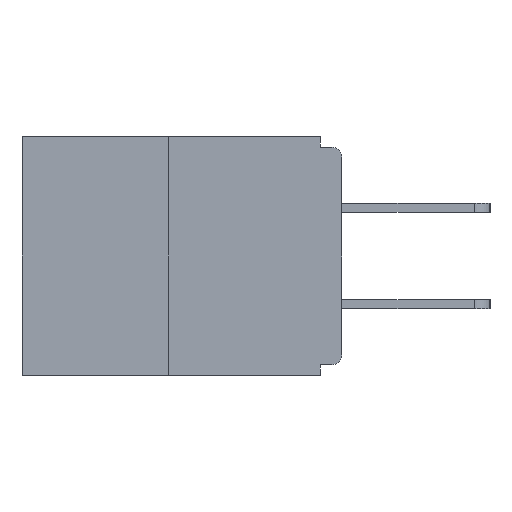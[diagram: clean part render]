
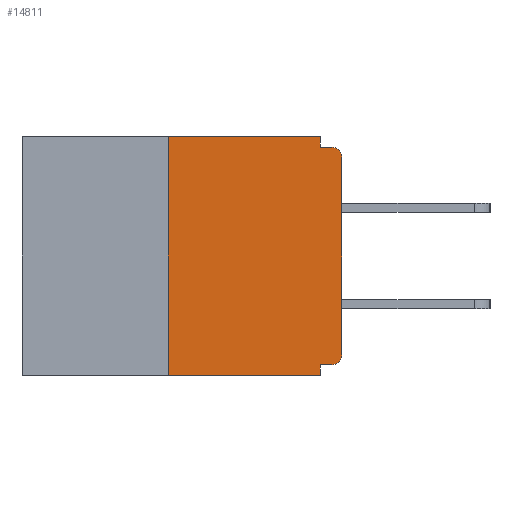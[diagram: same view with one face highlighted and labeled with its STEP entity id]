
A CAD part, left-side view. The second image highlights one B-rep face of the part: STEP entity #14811.
In plain terms, the highlighted planar face has unit normal (-1, 0, 0).
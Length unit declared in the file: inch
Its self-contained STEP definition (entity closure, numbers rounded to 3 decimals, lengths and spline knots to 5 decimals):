
#341 = EDGE_CURVE ( 'NONE', #14174, #8552, #1173, .T. ) ;
#707 = DIRECTION ( 'NONE',  ( 0., -1., 0. ) ) ;
#880 = ORIENTED_EDGE ( 'NONE', *, *, #341, .T. ) ;
#1102 = CARTESIAN_POINT ( 'NONE',  ( 0., 0.46, 0. ) ) ;
#1124 = DIRECTION ( 'NONE',  ( -1., 0., 0. ) ) ;
#1173 = CIRCLE ( 'NONE', #8427, 0.015 ) ;
#1279 = CIRCLE ( 'NONE', #10264, 0.015 ) ;
#1288 = ORIENTED_EDGE ( 'NONE', *, *, #7465, .T. ) ;
#2062 = CARTESIAN_POINT ( 'NONE',  ( 0., 0.25, 0. ) ) ;
#2180 = DIRECTION ( 'NONE',  ( 0., 0., -1. ) ) ;
#2292 = CARTESIAN_POINT ( 'NONE',  ( 0., 0.46, 0. ) ) ;
#2554 = CARTESIAN_POINT ( 'NONE',  ( 0., 0., 0. ) ) ;
#2937 = CARTESIAN_POINT ( 'NONE',  ( 0., 0.031, 0. ) ) ;
#3045 = LINE ( 'NONE', #2554, #7253 ) ;
#3136 = CARTESIAN_POINT ( 'NONE',  ( 0., 0.46, -0.343 ) ) ;
#3479 = LINE ( 'NONE', #16419, #13232 ) ;
#3625 = CARTESIAN_POINT ( 'NONE',  ( 0., 0.015, -0.015 ) ) ;
#3666 = DIRECTION ( 'NONE',  ( 0., 0., -1. ) ) ;
#3782 = CARTESIAN_POINT ( 'NONE',  ( 0., 0.015, -0.313 ) ) ;
#3856 = DIRECTION ( 'NONE',  ( 0., 0., 1. ) ) ;
#3902 = VERTEX_POINT ( 'NONE', #15123 ) ;
#4076 = EDGE_CURVE ( 'NONE', #8960, #9336, #14399, .T. ) ;
#4506 = DIRECTION ( 'NONE',  ( 0., -1., 0. ) ) ;
#4592 = EDGE_CURVE ( 'NONE', #7053, #8552, #11585, .T. ) ;
#4997 = PLANE ( 'NONE',  #16211 ) ;
#5063 = FACE_OUTER_BOUND ( 'NONE', #15114, .T. ) ;
#5150 = VERTEX_POINT ( 'NONE', #14991 ) ;
#5165 = CARTESIAN_POINT ( 'NONE',  ( 0., 0.25, 0. ) ) ;
#5410 = EDGE_CURVE ( 'NONE', #5150, #14174, #3045, .T. ) ;
#5808 = EDGE_CURVE ( 'NONE', #12360, #8960, #14711, .T. ) ;
#5948 = VERTEX_POINT ( 'NONE', #15202 ) ;
#6008 = CARTESIAN_POINT ( 'NONE',  ( 0., 0., -0.328 ) ) ;
#6629 = VERTEX_POINT ( 'NONE', #14404 ) ;
#6917 = EDGE_CURVE ( 'NONE', #6629, #3902, #3479, .T. ) ;
#7018 = EDGE_CURVE ( 'NONE', #5948, #5150, #1279, .T. ) ;
#7053 = VERTEX_POINT ( 'NONE', #7531 ) ;
#7224 = EDGE_CURVE ( 'NONE', #9336, #7053, #13584, .T. ) ;
#7253 = VECTOR ( 'NONE', #3856, 39.37008 ) ;
#7378 = DIRECTION ( 'NONE',  ( 0., 1., 0. ) ) ;
#7448 = CARTESIAN_POINT ( 'NONE',  ( 0., 0., -0.03 ) ) ;
#7465 = EDGE_CURVE ( 'NONE', #12360, #3902, #15368, .T. ) ;
#7504 = VECTOR ( 'NONE', #14130, 39.37008 ) ;
#7531 = CARTESIAN_POINT ( 'NONE',  ( 0., 0.031, -0.015 ) ) ;
#7771 = ORIENTED_EDGE ( 'NONE', *, *, #7018, .T. ) ;
#7797 = ORIENTED_EDGE ( 'NONE', *, *, #7224, .F. ) ;
#8427 = AXIS2_PLACEMENT_3D ( 'NONE', #12504, #1124, #2180 ) ;
#8552 = VERTEX_POINT ( 'NONE', #3625 ) ;
#8960 = VERTEX_POINT ( 'NONE', #5165 ) ;
#9336 = VERTEX_POINT ( 'NONE', #2937 ) ;
#9539 = VECTOR ( 'NONE', #707, 39.37008 ) ;
#9645 = CARTESIAN_POINT ( 'NONE',  ( 0., 0., -0.015 ) ) ;
#9994 = ORIENTED_EDGE ( 'NONE', *, *, #6917, .F. ) ;
#10100 = CARTESIAN_POINT ( 'NONE',  ( 0., 0.25, -0.343 ) ) ;
#10264 = AXIS2_PLACEMENT_3D ( 'NONE', #3782, #15272, #12943 ) ;
#11237 = DIRECTION ( 'NONE',  ( 0., 0., -1. ) ) ;
#11585 = LINE ( 'NONE', #9645, #13567 ) ;
#12360 = VERTEX_POINT ( 'NONE', #10100 ) ;
#12504 = CARTESIAN_POINT ( 'NONE',  ( 0., 0.015, -0.03 ) ) ;
#12943 = DIRECTION ( 'NONE',  ( 0., 0., -1. ) ) ;
#13232 = VECTOR ( 'NONE', #11237, 39.37008 ) ;
#13520 = VECTOR ( 'NONE', #14925, 39.37008 ) ;
#13547 = LINE ( 'NONE', #6008, #16379 ) ;
#13567 = VECTOR ( 'NONE', #4506, 39.37008 ) ;
#13584 = LINE ( 'NONE', #14018, #15382 ) ;
#14018 = CARTESIAN_POINT ( 'NONE',  ( 0., 0.031, 0. ) ) ;
#14130 = DIRECTION ( 'NONE',  ( 0., -1., 0. ) ) ;
#14174 = VERTEX_POINT ( 'NONE', #7448 ) ;
#14197 = ORIENTED_EDGE ( 'NONE', *, *, #5808, .F. ) ;
#14399 = LINE ( 'NONE', #1102, #7504 ) ;
#14404 = CARTESIAN_POINT ( 'NONE',  ( 0., 0.031, -0.328 ) ) ;
#14551 = ORIENTED_EDGE ( 'NONE', *, *, #4592, .F. ) ;
#14711 = LINE ( 'NONE', #2062, #13520 ) ;
#14811 = ADVANCED_FACE ( 'NONE', ( #5063 ), #4997, .F. ) ;
#14925 = DIRECTION ( 'NONE',  ( 0., 0., 1. ) ) ;
#14991 = CARTESIAN_POINT ( 'NONE',  ( 0., 0., -0.313 ) ) ;
#15114 = EDGE_LOOP ( 'NONE', ( #15829, #14197, #1288, #9994, #15162, #7771, #16373, #880, #14551, #7797 ) ) ;
#15123 = CARTESIAN_POINT ( 'NONE',  ( 0., 0.031, -0.343 ) ) ;
#15162 = ORIENTED_EDGE ( 'NONE', *, *, #16069, .F. ) ;
#15202 = CARTESIAN_POINT ( 'NONE',  ( 0., 0.015, -0.328 ) ) ;
#15272 = DIRECTION ( 'NONE',  ( -1., 0., 0. ) ) ;
#15318 = DIRECTION ( 'NONE',  ( 0., 0., -1. ) ) ;
#15368 = LINE ( 'NONE', #3136, #9539 ) ;
#15382 = VECTOR ( 'NONE', #15318, 39.37008 ) ;
#15829 = ORIENTED_EDGE ( 'NONE', *, *, #4076, .F. ) ;
#16069 = EDGE_CURVE ( 'NONE', #5948, #6629, #13547, .T. ) ;
#16211 = AXIS2_PLACEMENT_3D ( 'NONE', #2292, #16538, #3666 ) ;
#16373 = ORIENTED_EDGE ( 'NONE', *, *, #5410, .T. ) ;
#16379 = VECTOR ( 'NONE', #7378, 39.37008 ) ;
#16419 = CARTESIAN_POINT ( 'NONE',  ( 0., 0.031, -0.343 ) ) ;
#16538 = DIRECTION ( 'NONE',  ( 1., 0., 0. ) ) ;
